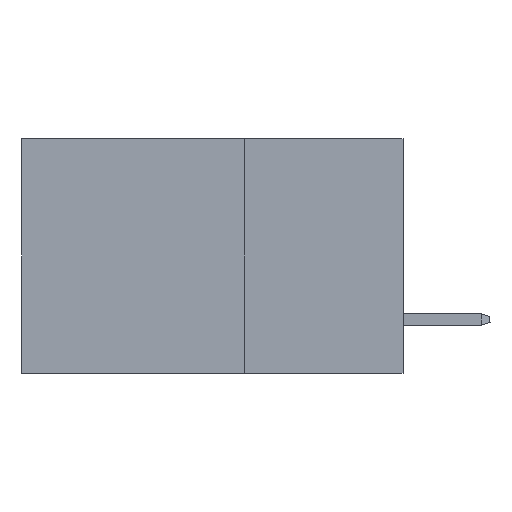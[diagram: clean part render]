
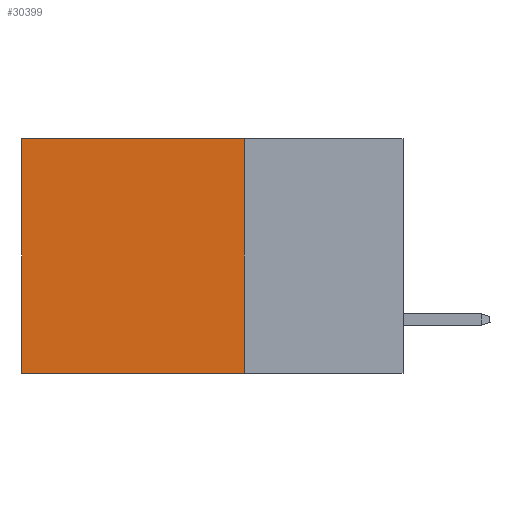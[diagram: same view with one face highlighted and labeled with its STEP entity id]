
A CAD part, left-side view. The second image highlights one B-rep face of the part: STEP entity #30399.
In plain terms, the highlighted planar face has unit normal (-1, 0, 0).
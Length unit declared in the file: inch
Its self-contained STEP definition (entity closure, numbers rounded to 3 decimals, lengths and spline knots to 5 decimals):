
#3326 = EDGE_CURVE ( 'NONE', #40133, #48709, #38949, .T. ) ;
#4107 = EDGE_CURVE ( 'NONE', #14043, #45491, #25007, .T. ) ;
#4155 = CARTESIAN_POINT ( 'NONE',  ( 0.2875, 0.25, 0. ) ) ;
#4418 = DIRECTION ( 'NONE',  ( 0., 1., 0. ) ) ;
#7104 = CARTESIAN_POINT ( 'NONE',  ( 0.2875, 0.25, 0. ) ) ;
#7272 = ORIENTED_EDGE ( 'NONE', *, *, #10151, .T. ) ;
#10151 = EDGE_CURVE ( 'NONE', #48709, #45491, #28351, .T. ) ;
#10641 = DIRECTION ( 'NONE',  ( 0., 0., -1. ) ) ;
#11147 = ORIENTED_EDGE ( 'NONE', *, *, #3326, .T. ) ;
#13605 = DIRECTION ( 'NONE',  ( 0., 0., -1. ) ) ;
#14043 = VERTEX_POINT ( 'NONE', #45321 ) ;
#15964 = CARTESIAN_POINT ( 'NONE',  ( 0.2875, 0.6, -0.37 ) ) ;
#18002 = LINE ( 'NONE', #7104, #20157 ) ;
#19404 = CARTESIAN_POINT ( 'NONE',  ( 0.2875, 0.25, 0. ) ) ;
#19638 = VECTOR ( 'NONE', #4418, 39.37008 ) ;
#20157 = VECTOR ( 'NONE', #10641, 39.37008 ) ;
#21668 = ORIENTED_EDGE ( 'NONE', *, *, #49123, .F. ) ;
#21698 = CARTESIAN_POINT ( 'NONE',  ( 0.2875, 0.25, -0.37 ) ) ;
#25007 = LINE ( 'NONE', #21698, #30234 ) ;
#26925 = EDGE_LOOP ( 'NONE', ( #7272, #46479, #21668, #11147 ) ) ;
#28351 = LINE ( 'NONE', #48448, #30170 ) ;
#30170 = VECTOR ( 'NONE', #13605, 39.37008 ) ;
#30234 = VECTOR ( 'NONE', #32901, 39.37008 ) ;
#30399 = ADVANCED_FACE ( 'NONE', ( #43297 ), #42545, .F. ) ;
#32901 = DIRECTION ( 'NONE',  ( 0., 1., 0. ) ) ;
#35159 = DIRECTION ( 'NONE',  ( 1., 0., 0. ) ) ;
#38725 = DIRECTION ( 'NONE',  ( 0., 0., -1. ) ) ;
#38949 = LINE ( 'NONE', #4155, #19638 ) ;
#40133 = VERTEX_POINT ( 'NONE', #47903 ) ;
#41205 = CARTESIAN_POINT ( 'NONE',  ( 0.2875, 0.6, 0. ) ) ;
#42545 = PLANE ( 'NONE',  #43096 ) ;
#43096 = AXIS2_PLACEMENT_3D ( 'NONE', #19404, #35159, #38725 ) ;
#43297 = FACE_OUTER_BOUND ( 'NONE', #26925, .T. ) ;
#45321 = CARTESIAN_POINT ( 'NONE',  ( 0.2875, 0.25, -0.37 ) ) ;
#45491 = VERTEX_POINT ( 'NONE', #15964 ) ;
#46479 = ORIENTED_EDGE ( 'NONE', *, *, #4107, .F. ) ;
#47903 = CARTESIAN_POINT ( 'NONE',  ( 0.2875, 0.25, 0. ) ) ;
#48448 = CARTESIAN_POINT ( 'NONE',  ( 0.2875, 0.6, 0. ) ) ;
#48709 = VERTEX_POINT ( 'NONE', #41205 ) ;
#49123 = EDGE_CURVE ( 'NONE', #40133, #14043, #18002, .T. ) ;
